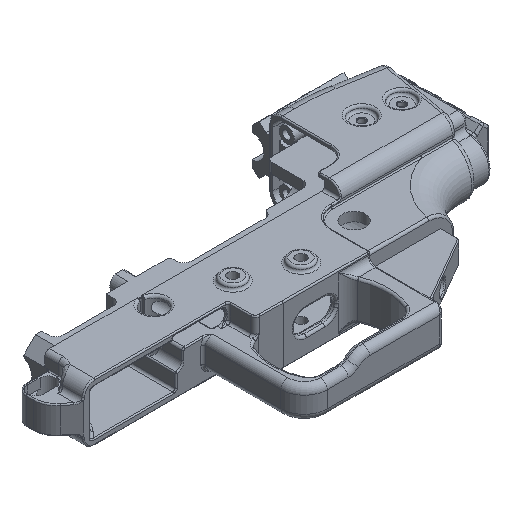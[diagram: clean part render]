
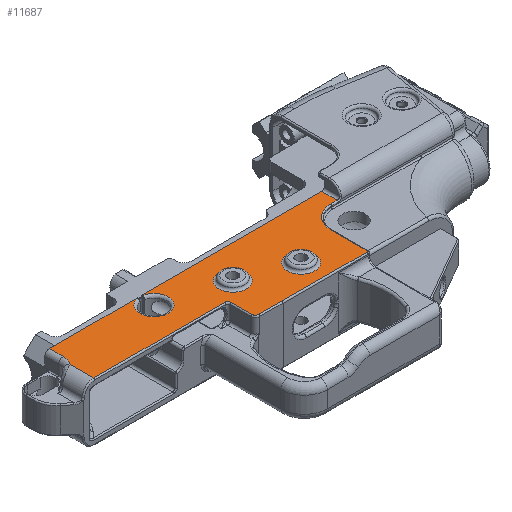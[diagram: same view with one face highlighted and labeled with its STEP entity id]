
A CAD part, isometric view. The second image highlights one B-rep face of the part: STEP entity #11687.
In plain terms, the highlighted face is planar.
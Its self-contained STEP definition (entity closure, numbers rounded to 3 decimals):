
#240=FACE_BOUND('',#1334,.T.);
#241=FACE_BOUND('',#1335,.T.);
#290=PLANE('',#12454);
#606=FACE_OUTER_BOUND('',#1333,.T.);
#1333=EDGE_LOOP('',(#7765,#7766,#7767,#7768,#7769,#7770,#7771,#7772,#7773,
#7774,#7775,#7776,#7777,#7778,#7779,#7780,#7781,#7782,#7783));
#1334=EDGE_LOOP('',(#7784));
#1335=EDGE_LOOP('',(#7785));
#2285=LINE('',#17898,#3166);
#2286=LINE('',#17900,#3167);
#2287=LINE('',#17904,#3168);
#2288=LINE('',#17906,#3169);
#2289=LINE('',#17910,#3170);
#2290=LINE('',#17914,#3171);
#2291=LINE('',#17916,#3172);
#2292=LINE('',#17920,#3173);
#2293=LINE('',#17924,#3174);
#2294=LINE('',#17926,#3175);
#2295=LINE('',#17928,#3176);
#3166=VECTOR('',#13912,39.75);
#3167=VECTOR('',#13913,10.);
#3168=VECTOR('',#13916,10.);
#3169=VECTOR('',#13917,10.);
#3170=VECTOR('',#13920,10.);
#3171=VECTOR('',#13923,10.);
#3172=VECTOR('',#13924,10.);
#3173=VECTOR('',#13927,10.);
#3174=VECTOR('',#13930,10.);
#3175=VECTOR('',#13931,10.);
#3176=VECTOR('',#13932,10.);
#4062=CIRCLE('',#12453,6.);
#4063=CIRCLE('',#12455,6.125);
#4064=CIRCLE('',#12456,0.5);
#4065=CIRCLE('',#12457,6.47);
#4066=CIRCLE('',#12458,1.5);
#4067=CIRCLE('',#12459,1.5);
#4068=CIRCLE('',#12460,0.5);
#4069=CIRCLE('',#12461,9.5);
#4070=CIRCLE('',#12462,0.5);
#4071=CIRCLE('',#12463,6.);
#4783=VERTEX_POINT('',#17888);
#4784=VERTEX_POINT('',#17892);
#4785=VERTEX_POINT('',#17893);
#4786=VERTEX_POINT('',#17895);
#4787=VERTEX_POINT('',#17897);
#4788=VERTEX_POINT('',#17899);
#4789=VERTEX_POINT('',#17901);
#4790=VERTEX_POINT('',#17903);
#4791=VERTEX_POINT('',#17905);
#4792=VERTEX_POINT('',#17907);
#4793=VERTEX_POINT('',#17909);
#4794=VERTEX_POINT('',#17911);
#4795=VERTEX_POINT('',#17913);
#4796=VERTEX_POINT('',#17915);
#4797=VERTEX_POINT('',#17917);
#4798=VERTEX_POINT('',#17919);
#4799=VERTEX_POINT('',#17921);
#4800=VERTEX_POINT('',#17923);
#4801=VERTEX_POINT('',#17925);
#4802=VERTEX_POINT('',#17927);
#4803=VERTEX_POINT('',#17930);
#5911=EDGE_CURVE('',#4783,#4783,#4062,.T.);
#5912=EDGE_CURVE('',#4784,#4785,#4063,.T.);
#5913=EDGE_CURVE('',#4784,#4786,#4064,.T.);
#5914=EDGE_CURVE('',#4787,#4786,#2285,.T.);
#5915=EDGE_CURVE('',#4788,#4787,#2286,.T.);
#5916=EDGE_CURVE('',#4789,#4788,#4065,.T.);
#5917=EDGE_CURVE('',#4790,#4789,#2287,.T.);
#5918=EDGE_CURVE('',#4791,#4790,#2288,.T.);
#5919=EDGE_CURVE('',#4792,#4791,#4066,.T.);
#5920=EDGE_CURVE('',#4793,#4792,#2289,.T.);
#5921=EDGE_CURVE('',#4794,#4793,#4067,.T.);
#5922=EDGE_CURVE('',#4795,#4794,#2290,.T.);
#5923=EDGE_CURVE('',#4796,#4795,#2291,.T.);
#5924=EDGE_CURVE('',#4797,#4796,#4068,.T.);
#5925=EDGE_CURVE('',#4798,#4797,#2292,.T.);
#5926=EDGE_CURVE('',#4799,#4798,#4069,.T.);
#5927=EDGE_CURVE('',#4800,#4799,#2293,.T.);
#5928=EDGE_CURVE('',#4801,#4800,#2294,.T.);
#5929=EDGE_CURVE('',#4802,#4801,#2295,.T.);
#5930=EDGE_CURVE('',#4802,#4785,#4070,.T.);
#5931=EDGE_CURVE('',#4803,#4803,#4071,.T.);
#7765=ORIENTED_EDGE('',*,*,#5912,.F.);
#7766=ORIENTED_EDGE('',*,*,#5913,.T.);
#7767=ORIENTED_EDGE('',*,*,#5914,.F.);
#7768=ORIENTED_EDGE('',*,*,#5915,.F.);
#7769=ORIENTED_EDGE('',*,*,#5916,.F.);
#7770=ORIENTED_EDGE('',*,*,#5917,.F.);
#7771=ORIENTED_EDGE('',*,*,#5918,.F.);
#7772=ORIENTED_EDGE('',*,*,#5919,.F.);
#7773=ORIENTED_EDGE('',*,*,#5920,.F.);
#7774=ORIENTED_EDGE('',*,*,#5921,.F.);
#7775=ORIENTED_EDGE('',*,*,#5922,.F.);
#7776=ORIENTED_EDGE('',*,*,#5923,.F.);
#7777=ORIENTED_EDGE('',*,*,#5924,.F.);
#7778=ORIENTED_EDGE('',*,*,#5925,.F.);
#7779=ORIENTED_EDGE('',*,*,#5926,.F.);
#7780=ORIENTED_EDGE('',*,*,#5927,.F.);
#7781=ORIENTED_EDGE('',*,*,#5928,.F.);
#7782=ORIENTED_EDGE('',*,*,#5929,.F.);
#7783=ORIENTED_EDGE('',*,*,#5930,.T.);
#7784=ORIENTED_EDGE('',*,*,#5931,.F.);
#7785=ORIENTED_EDGE('',*,*,#5911,.F.);
#11687=ADVANCED_FACE('',(#606,#240,#241),#290,.T.);
#12453=AXIS2_PLACEMENT_3D('',#17890,#13904,#13905);
#12454=AXIS2_PLACEMENT_3D('',#17891,#13906,#13907);
#12455=AXIS2_PLACEMENT_3D('',#17894,#13908,#13909);
#12456=AXIS2_PLACEMENT_3D('',#17896,#13910,#13911);
#12457=AXIS2_PLACEMENT_3D('',#17902,#13914,#13915);
#12458=AXIS2_PLACEMENT_3D('',#17908,#13918,#13919);
#12459=AXIS2_PLACEMENT_3D('',#17912,#13921,#13922);
#12460=AXIS2_PLACEMENT_3D('',#17918,#13925,#13926);
#12461=AXIS2_PLACEMENT_3D('',#17922,#13928,#13929);
#12462=AXIS2_PLACEMENT_3D('',#17929,#13933,#13934);
#12463=AXIS2_PLACEMENT_3D('',#17931,#13935,#13936);
#13904=DIRECTION('center_axis',(0.,0.,-1.));
#13905=DIRECTION('ref_axis',(1.,0.,0.));
#13906=DIRECTION('center_axis',(0.,0.,-1.));
#13907=DIRECTION('ref_axis',(1.,0.,0.));
#13908=DIRECTION('center_axis',(0.,0.,-1.));
#13909=DIRECTION('ref_axis',(0.,-1.,0.));
#13910=DIRECTION('center_axis',(0.,0.,1.));
#13911=DIRECTION('ref_axis',(0.707,0.707,0.));
#13912=DIRECTION('',(-1.,0.,0.));
#13913=DIRECTION('',(0.,1.,0.));
#13914=DIRECTION('center_axis',(0.,0.,-1.));
#13915=DIRECTION('ref_axis',(-1.,0.,0.));
#13916=DIRECTION('',(0.,1.,0.));
#13917=DIRECTION('',(1.,0.,0.));
#13918=DIRECTION('center_axis',(0.,0.,-1.));
#13919=DIRECTION('ref_axis',(-0.707,0.707,0.));
#13920=DIRECTION('',(0.,1.,0.));
#13921=DIRECTION('center_axis',(0.,0.,1.));
#13922=DIRECTION('ref_axis',(0.71,-0.704,0.));
#13923=DIRECTION('',(1.,0.008,0.));
#13924=DIRECTION('',(1.,0.,0.));
#13925=DIRECTION('center_axis',(0.,0.,1.));
#13926=DIRECTION('ref_axis',(-0.707,-0.707,0.));
#13927=DIRECTION('',(0.,-1.,0.));
#13928=DIRECTION('center_axis',(0.,0.,-1.));
#13929=DIRECTION('ref_axis',(0.707,0.707,0.));
#13930=DIRECTION('',(1.,0.,0.));
#13931=DIRECTION('',(0.,-1.,0.));
#13932=DIRECTION('',(-1.,0.,0.));
#13933=DIRECTION('center_axis',(0.,0.,1.));
#13934=DIRECTION('ref_axis',(-0.707,0.707,0.));
#13935=DIRECTION('center_axis',(0.,0.,-1.));
#13936=DIRECTION('ref_axis',(1.,0.,0.));
#17888=CARTESIAN_POINT('',(79.954,6.799,-12.457));
#17890=CARTESIAN_POINT('Origin',(85.954,6.799,-12.457));
#17891=CARTESIAN_POINT('Origin',(83.274,-108.44,-12.457));
#17892=CARTESIAN_POINT('',(112.98,20.776,-12.457));
#17893=CARTESIAN_POINT('',(110.999,20.776,-12.457));
#17894=CARTESIAN_POINT('Origin',(111.989,14.732,-12.457));
#17895=CARTESIAN_POINT('',(112.917,21.019,-12.457));
#17896=CARTESIAN_POINT('Origin',(112.48,20.776,-12.457));
#17897=CARTESIAN_POINT('',(150.73,21.019,-12.457));
#17898=CARTESIAN_POINT('',(152.73,21.019,-12.457));
#17899=CARTESIAN_POINT('',(150.73,15.088,-12.457));
#17900=CARTESIAN_POINT('',(150.73,-39.183,-12.457));
#17901=CARTESIAN_POINT('',(152.201,10.981,-12.457));
#17902=CARTESIAN_POINT('Origin',(157.201,15.088,-12.457));
#17903=CARTESIAN_POINT('',(152.201,0.5,-12.457));
#17904=CARTESIAN_POINT('',(152.201,-48.911,-12.457));
#17905=CARTESIAN_POINT('',(95.882,0.5,-12.457));
#17906=CARTESIAN_POINT('',(41.637,0.5,-12.457));
#17907=CARTESIAN_POINT('',(94.382,-1.,-12.457));
#17908=CARTESIAN_POINT('Origin',(95.882,-1.,-12.457));
#17909=CARTESIAN_POINT('',(94.382,-9.796,-12.457));
#17910=CARTESIAN_POINT('',(94.382,-54.22,-12.457));
#17911=CARTESIAN_POINT('',(92.893,-11.296,-12.457));
#17912=CARTESIAN_POINT('Origin',(92.882,-9.796,-12.457));
#17913=CARTESIAN_POINT('',(83.007,-11.373,-12.457));
#17914=CARTESIAN_POINT('',(82.761,-11.375,-12.457));
#17915=CARTESIAN_POINT('',(46.306,-11.373,-12.457));
#17916=CARTESIAN_POINT('',(83.141,-11.373,-12.457));
#17917=CARTESIAN_POINT('',(45.806,-10.873,-12.457));
#17918=CARTESIAN_POINT('Origin',(46.306,-10.873,-12.457));
#17919=CARTESIAN_POINT('',(45.806,4.878,-12.457));
#17920=CARTESIAN_POINT('',(45.806,-60.157,-12.457));
#17921=CARTESIAN_POINT('',(36.306,14.378,-12.457));
#17922=CARTESIAN_POINT('Origin',(36.306,4.878,-12.457));
#17923=CARTESIAN_POINT('',(33.41,14.378,-12.457));
#17924=CARTESIAN_POINT('',(44.137,14.378,-12.457));
#17925=CARTESIAN_POINT('',(33.41,21.019,-12.457));
#17926=CARTESIAN_POINT('',(33.41,-108.44,-12.457));
#17927=CARTESIAN_POINT('',(111.061,21.019,-12.457));
#17928=CARTESIAN_POINT('',(81.026,21.019,-12.457));
#17929=CARTESIAN_POINT('Origin',(111.499,20.776,-12.457));
#17930=CARTESIAN_POINT('',(58.541,-1.177,-12.457));
#17931=CARTESIAN_POINT('Origin',(64.541,-1.177,-12.457));
